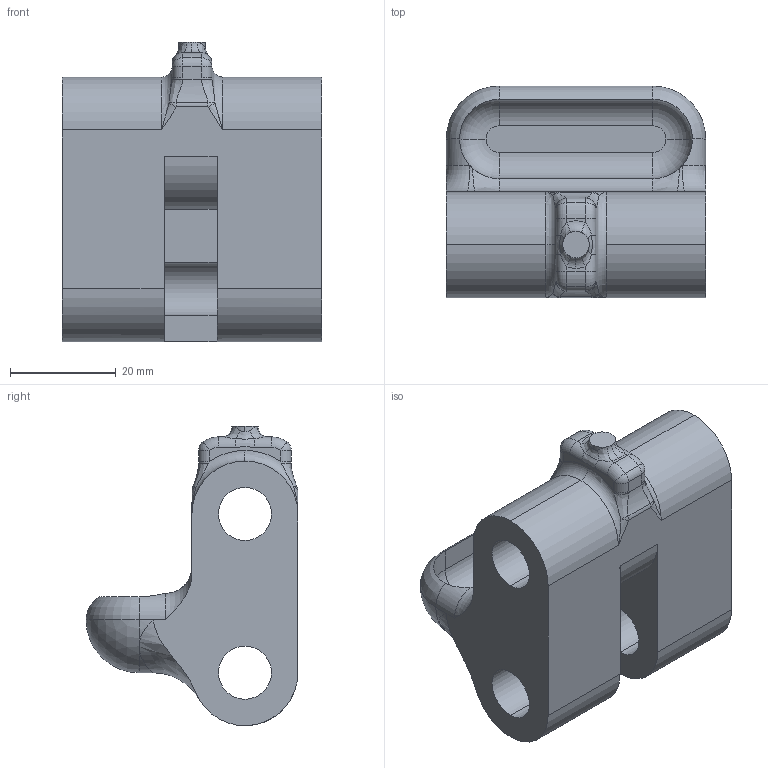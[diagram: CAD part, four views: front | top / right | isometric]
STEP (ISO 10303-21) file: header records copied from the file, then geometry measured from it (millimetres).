
FILE_DESCRIPTION (( 'STEP AP203' ), '1' );
FILE_NAME ('Hammer Slide.STEP', '2013-08-28T13:22:51', ( '' ), ( '' ), 'SwSTEP 2.0', 'SolidWorks 2013', '' );
FILE_SCHEMA (( 'CONFIG_CONTROL_DESIGN' ));
Length unit declared in the file: millimetre
Products named in the file (1): Hammer Slide
Bounding box: 49 x 40 x 56.56 mm (x, y, z)
Volume: 43110.8 mm3; surface area: 13485.9 mm2
Topology: 1 solids, 1 shells, 120 faces, 297 edges, 163 vertices
Faces by surface type: cylinder 45, bspline 26, plane 21, torus 18, sphere 10
Entity records: 4695 total; most frequent: CARTESIAN_POINT 2010, ORIENTED_EDGE 566, DIRECTION 536, EDGE_CURVE 283, AXIS2_PLACEMENT_3D 227, VERTEX_POINT 163, CIRCLE 132, EDGE_LOOP 124
